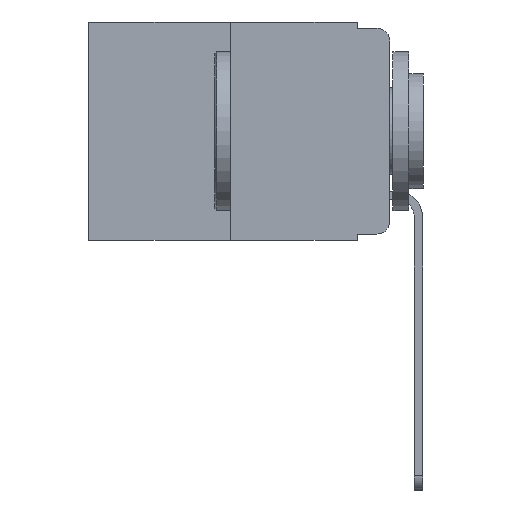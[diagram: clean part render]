
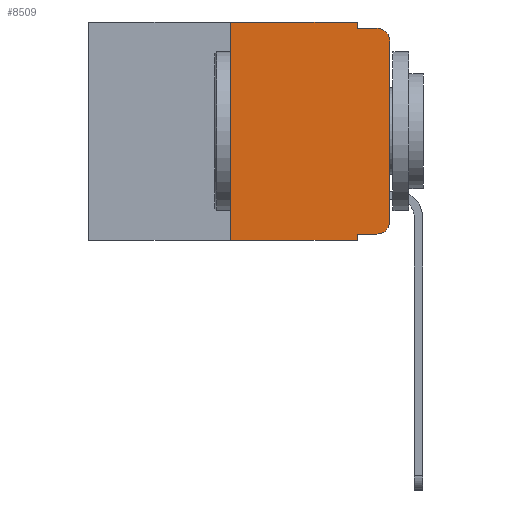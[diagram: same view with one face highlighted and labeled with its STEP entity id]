
A CAD part, left-side view. The second image highlights one B-rep face of the part: STEP entity #8509.
In plain terms, the highlighted planar face has unit normal (-1, 0, 0).
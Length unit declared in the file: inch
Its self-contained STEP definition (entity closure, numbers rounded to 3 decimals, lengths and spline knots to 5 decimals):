
#31 = EDGE_CURVE ( 'NONE', #1228, #3389, #6660, .T. ) ;
#34 = EDGE_CURVE ( 'NONE', #3389, #1637, #9568, .T. ) ;
#450 = DIRECTION ( 'NONE',  ( 0., -1., 0. ) ) ;
#822 = VERTEX_POINT ( 'NONE', #4643 ) ;
#928 = DIRECTION ( 'NONE',  ( 0., 0., -1. ) ) ;
#1228 = VERTEX_POINT ( 'NONE', #3281 ) ;
#1354 = VECTOR ( 'NONE', #2897, 39.37008 ) ;
#1637 = VERTEX_POINT ( 'NONE', #6189 ) ;
#1639 = VERTEX_POINT ( 'NONE', #6172 ) ;
#1700 = DIRECTION ( 'NONE',  ( 0., 0., -1. ) ) ;
#2132 = CARTESIAN_POINT ( 'NONE',  ( 0., 0.051, -0.01 ) ) ;
#2535 = VERTEX_POINT ( 'NONE', #3024 ) ;
#2648 = LINE ( 'NONE', #2132, #7983 ) ;
#2758 = AXIS2_PLACEMENT_3D ( 'NONE', #9883, #12060, #12043 ) ;
#2897 = DIRECTION ( 'NONE',  ( 0., -1., 0. ) ) ;
#2984 = VERTEX_POINT ( 'NONE', #12710 ) ;
#3024 = CARTESIAN_POINT ( 'NONE',  ( 0., 0.25, -0.343 ) ) ;
#3278 = DIRECTION ( 'NONE',  ( 0., -1., 0. ) ) ;
#3281 = CARTESIAN_POINT ( 'NONE',  ( 0., 0.051, -0.333 ) ) ;
#3386 = LINE ( 'NONE', #10339, #5963 ) ;
#3389 = VERTEX_POINT ( 'NONE', #7578 ) ;
#3761 = FACE_OUTER_BOUND ( 'NONE', #3779, .T. ) ;
#3779 = EDGE_LOOP ( 'NONE', ( #5057, #5181, #5463, #5636, #5666, #6114, #6153, #6427, #6442, #6580 ) ) ;
#3800 = VECTOR ( 'NONE', #450, 39.37008 ) ;
#4081 = DIRECTION ( 'NONE',  ( 1., 0., 0. ) ) ;
#4112 = CARTESIAN_POINT ( 'NONE',  ( 0., 0.25, 0. ) ) ;
#4642 = CARTESIAN_POINT ( 'NONE',  ( 0., 0.25, 0. ) ) ;
#4643 = CARTESIAN_POINT ( 'NONE',  ( 0., 0.051, -0.01 ) ) ;
#4670 = LINE ( 'NONE', #7704, #9691 ) ;
#4985 = VECTOR ( 'NONE', #928, 39.37008 ) ;
#5057 = ORIENTED_EDGE ( 'NONE', *, *, #13358, .T. ) ;
#5139 = CARTESIAN_POINT ( 'NONE',  ( 0., 0.051, -0.343 ) ) ;
#5181 = ORIENTED_EDGE ( 'NONE', *, *, #13375, .T. ) ;
#5432 = VERTEX_POINT ( 'NONE', #4112 ) ;
#5451 = DIRECTION ( 'NONE',  ( 0., 0., 1. ) ) ;
#5463 = ORIENTED_EDGE ( 'NONE', *, *, #13387, .F. ) ;
#5493 = CARTESIAN_POINT ( 'NONE',  ( 0., 0.02, -0.03 ) ) ;
#5636 = ORIENTED_EDGE ( 'NONE', *, *, #13406, .F. ) ;
#5666 = ORIENTED_EDGE ( 'NONE', *, *, #8086, .F. ) ;
#5963 = VECTOR ( 'NONE', #5451, 39.37008 ) ;
#6114 = ORIENTED_EDGE ( 'NONE', *, *, #10024, .F. ) ;
#6153 = ORIENTED_EDGE ( 'NONE', *, *, #12903, .T. ) ;
#6172 = CARTESIAN_POINT ( 'NONE',  ( 0., 0.02, -0.01 ) ) ;
#6189 = CARTESIAN_POINT ( 'NONE',  ( 0., 0., -0.313 ) ) ;
#6427 = ORIENTED_EDGE ( 'NONE', *, *, #8652, .F. ) ;
#6442 = ORIENTED_EDGE ( 'NONE', *, *, #31, .T. ) ;
#6504 = DIRECTION ( 'NONE',  ( 0., 0., -1. ) ) ;
#6580 = ORIENTED_EDGE ( 'NONE', *, *, #34, .T. ) ;
#6617 = LINE ( 'NONE', #8636, #11451 ) ;
#6660 = LINE ( 'NONE', #13524, #3800 ) ;
#6696 = AXIS2_PLACEMENT_3D ( 'NONE', #5493, #12321, #6504 ) ;
#6825 = CARTESIAN_POINT ( 'NONE',  ( 0., 0.473, 0. ) ) ;
#7578 = CARTESIAN_POINT ( 'NONE',  ( 0., 0.02, -0.333 ) ) ;
#7704 = CARTESIAN_POINT ( 'NONE',  ( 0., 0.473, 0. ) ) ;
#7983 = VECTOR ( 'NONE', #3278, 39.37008 ) ;
#8086 = EDGE_CURVE ( 'NONE', #5432, #2984, #4670, .T. ) ;
#8090 = CARTESIAN_POINT ( 'NONE',  ( 0., 0., -0.03 ) ) ;
#8509 = ADVANCED_FACE ( 'NONE', ( #3761 ), #9118, .F. ) ;
#8636 = CARTESIAN_POINT ( 'NONE',  ( 0., 0.051, 0. ) ) ;
#8652 = EDGE_CURVE ( 'NONE', #1228, #9903, #6617, .T. ) ;
#9036 = VECTOR ( 'NONE', #11536, 39.37008 ) ;
#9118 = PLANE ( 'NONE',  #12667 ) ;
#9135 = CARTESIAN_POINT ( 'NONE',  ( 0., 0.473, -0.343 ) ) ;
#9568 = CIRCLE ( 'NONE', #2758, 0.02 ) ;
#9691 = VECTOR ( 'NONE', #9710, 39.37008 ) ;
#9710 = DIRECTION ( 'NONE',  ( 0., -1., 0. ) ) ;
#9883 = CARTESIAN_POINT ( 'NONE',  ( 0., 0.02, -0.313 ) ) ;
#9903 = VERTEX_POINT ( 'NONE', #5139 ) ;
#10024 = EDGE_CURVE ( 'NONE', #2535, #5432, #11580, .T. ) ;
#10339 = CARTESIAN_POINT ( 'NONE',  ( 0., 0., 0. ) ) ;
#11150 = CIRCLE ( 'NONE', #6696, 0.02 ) ;
#11451 = VECTOR ( 'NONE', #12531, 39.37008 ) ;
#11536 = DIRECTION ( 'NONE',  ( 0., 0., 1. ) ) ;
#11580 = LINE ( 'NONE', #4642, #9036 ) ;
#12043 = DIRECTION ( 'NONE',  ( 0., 0., -1. ) ) ;
#12060 = DIRECTION ( 'NONE',  ( -1., 0., 0. ) ) ;
#12249 = VERTEX_POINT ( 'NONE', #8090 ) ;
#12321 = DIRECTION ( 'NONE',  ( -1., 0., 0. ) ) ;
#12531 = DIRECTION ( 'NONE',  ( 0., 0., -1. ) ) ;
#12666 = LINE ( 'NONE', #9135, #1354 ) ;
#12667 = AXIS2_PLACEMENT_3D ( 'NONE', #6825, #4081, #1700 ) ;
#12710 = CARTESIAN_POINT ( 'NONE',  ( 0., 0.051, 0. ) ) ;
#12797 = LINE ( 'NONE', #13310, #4985 ) ;
#12903 = EDGE_CURVE ( 'NONE', #2535, #9903, #12666, .T. ) ;
#13310 = CARTESIAN_POINT ( 'NONE',  ( 0., 0.051, 0. ) ) ;
#13358 = EDGE_CURVE ( 'NONE', #1637, #12249, #3386, .T. ) ;
#13375 = EDGE_CURVE ( 'NONE', #12249, #1639, #11150, .T. ) ;
#13387 = EDGE_CURVE ( 'NONE', #822, #1639, #2648, .T. ) ;
#13406 = EDGE_CURVE ( 'NONE', #2984, #822, #12797, .T. ) ;
#13524 = CARTESIAN_POINT ( 'NONE',  ( 0., 0.051, -0.333 ) ) ;
